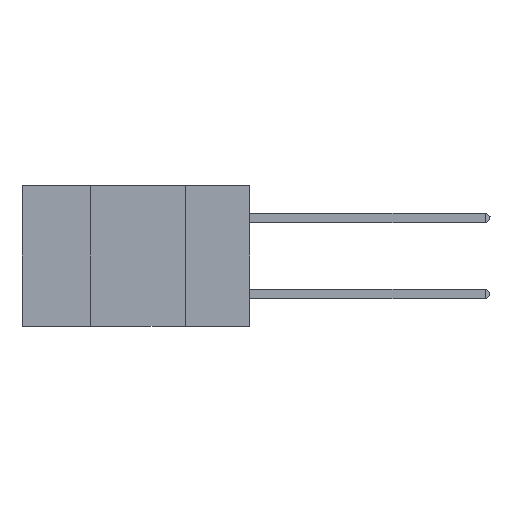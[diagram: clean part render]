
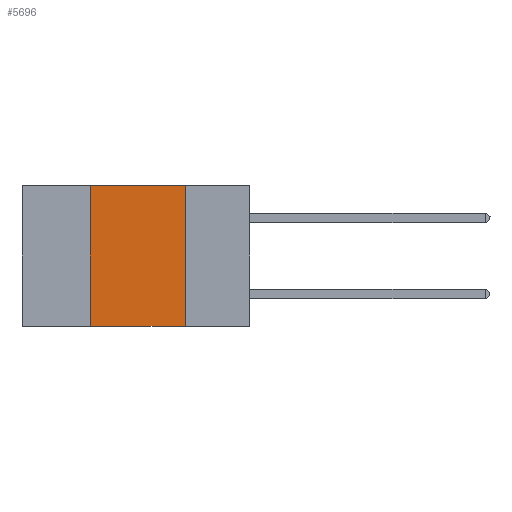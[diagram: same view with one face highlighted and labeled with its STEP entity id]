
A CAD part, left-side view. The second image highlights one B-rep face of the part: STEP entity #5696.
In plain terms, the highlighted planar face has unit normal (-1, 0, 0).
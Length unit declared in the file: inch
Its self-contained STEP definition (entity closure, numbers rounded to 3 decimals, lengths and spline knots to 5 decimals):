
#191 = CARTESIAN_POINT ( 'NONE',  ( 0., 0.42, 0. ) ) ;
#406 = AXIS2_PLACEMENT_3D ( 'NONE', #7659, #6838, #9993 ) ;
#573 = VERTEX_POINT ( 'NONE', #5360 ) ;
#608 = LINE ( 'NONE', #9122, #885 ) ;
#885 = VECTOR ( 'NONE', #4382, 39.37008 ) ;
#905 = FACE_OUTER_BOUND ( 'NONE', #9944, .T. ) ;
#1085 = VERTEX_POINT ( 'NONE', #1231 ) ;
#1231 = CARTESIAN_POINT ( 'NONE',  ( 0., 0.42, 0. ) ) ;
#1450 = ORIENTED_EDGE ( 'NONE', *, *, #3331, .F. ) ;
#1468 = EDGE_CURVE ( 'NONE', #4444, #573, #608, .T. ) ;
#1698 = CARTESIAN_POINT ( 'NONE',  ( 0., 0.17, 0. ) ) ;
#2125 = LINE ( 'NONE', #4832, #5151 ) ;
#2733 = EDGE_CURVE ( 'NONE', #7948, #573, #2125, .T. ) ;
#2989 = VECTOR ( 'NONE', #7417, 39.37008 ) ;
#3331 = EDGE_CURVE ( 'NONE', #4444, #1085, #8973, .T. ) ;
#3453 = PLANE ( 'NONE',  #406 ) ;
#3727 = ORIENTED_EDGE ( 'NONE', *, *, #1468, .T. ) ;
#3926 = LINE ( 'NONE', #9114, #8390 ) ;
#4382 = DIRECTION ( 'NONE',  ( 0., -1., 0. ) ) ;
#4444 = VERTEX_POINT ( 'NONE', #4731 ) ;
#4731 = CARTESIAN_POINT ( 'NONE',  ( 0., 0.42, -0.37 ) ) ;
#4832 = CARTESIAN_POINT ( 'NONE',  ( 0., 0.17, 0. ) ) ;
#5151 = VECTOR ( 'NONE', #7865, 39.37008 ) ;
#5360 = CARTESIAN_POINT ( 'NONE',  ( 0., 0.17, -0.37 ) ) ;
#5696 = ADVANCED_FACE ( 'NONE', ( #905 ), #3453, .F. ) ;
#6838 = DIRECTION ( 'NONE',  ( 1., 0., 0. ) ) ;
#7417 = DIRECTION ( 'NONE',  ( 0., 0., 1. ) ) ;
#7546 = EDGE_CURVE ( 'NONE', #1085, #7948, #3926, .T. ) ;
#7659 = CARTESIAN_POINT ( 'NONE',  ( 0., 0.6, 0. ) ) ;
#7865 = DIRECTION ( 'NONE',  ( 0., 0., -1. ) ) ;
#7948 = VERTEX_POINT ( 'NONE', #1698 ) ;
#8390 = VECTOR ( 'NONE', #9081, 39.37008 ) ;
#8768 = ORIENTED_EDGE ( 'NONE', *, *, #7546, .F. ) ;
#8973 = LINE ( 'NONE', #191, #2989 ) ;
#9081 = DIRECTION ( 'NONE',  ( 0., -1., 0. ) ) ;
#9114 = CARTESIAN_POINT ( 'NONE',  ( 0., 0.6, 0. ) ) ;
#9122 = CARTESIAN_POINT ( 'NONE',  ( 0., 0.6, -0.37 ) ) ;
#9534 = ORIENTED_EDGE ( 'NONE', *, *, #2733, .F. ) ;
#9944 = EDGE_LOOP ( 'NONE', ( #9534, #8768, #1450, #3727 ) ) ;
#9993 = DIRECTION ( 'NONE',  ( 0., 0., -1. ) ) ;
